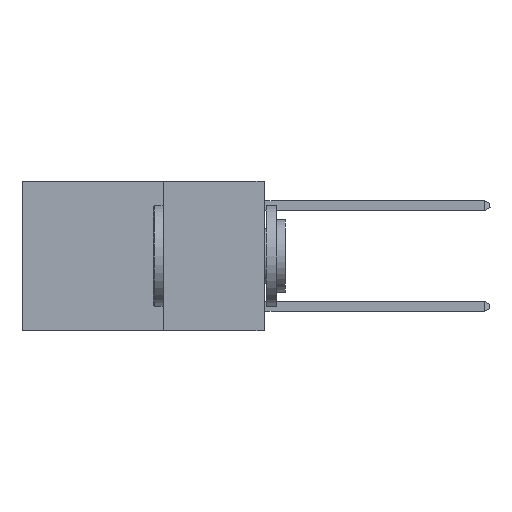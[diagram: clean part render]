
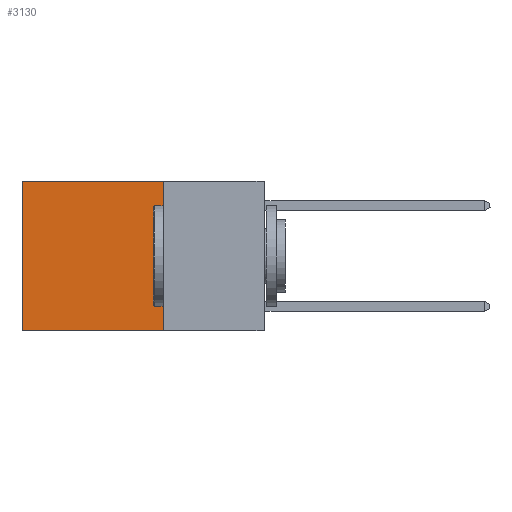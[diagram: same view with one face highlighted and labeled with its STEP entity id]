
A CAD part, left-side view. The second image highlights one B-rep face of the part: STEP entity #3130.
In plain terms, the highlighted planar face has unit normal (-1, 0, 0).
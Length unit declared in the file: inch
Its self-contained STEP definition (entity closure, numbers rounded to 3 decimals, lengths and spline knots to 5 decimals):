
#243 = VERTEX_POINT ( 'NONE', #12224 ) ;
#468 = DIRECTION ( 'NONE',  ( 0., 1., 0. ) ) ;
#2147 = PLANE ( 'NONE',  #14639 ) ;
#3090 = ORIENTED_EDGE ( 'NONE', *, *, #7713, .F. ) ;
#3130 = ADVANCED_FACE ( 'NONE', ( #13995 ), #2147, .F. ) ;
#3532 = ORIENTED_EDGE ( 'NONE', *, *, #5945, .T. ) ;
#3566 = DIRECTION ( 'NONE',  ( 1., 0., 0. ) ) ;
#4046 = LINE ( 'NONE', #7949, #10388 ) ;
#4439 = CARTESIAN_POINT ( 'NONE',  ( 0.2625, 0.6, 0. ) ) ;
#4689 = LINE ( 'NONE', #11690, #8244 ) ;
#5429 = EDGE_CURVE ( 'NONE', #16957, #13461, #14746, .T. ) ;
#5945 = EDGE_CURVE ( 'NONE', #243, #14178, #10211, .T. ) ;
#7367 = ORIENTED_EDGE ( 'NONE', *, *, #11386, .T. ) ;
#7713 = EDGE_CURVE ( 'NONE', #243, #16957, #4046, .T. ) ;
#7949 = CARTESIAN_POINT ( 'NONE',  ( 0.2625, 0.25, 0. ) ) ;
#8244 = VECTOR ( 'NONE', #14406, 39.37008 ) ;
#8345 = VECTOR ( 'NONE', #17150, 39.37008 ) ;
#9027 = ORIENTED_EDGE ( 'NONE', *, *, #5429, .F. ) ;
#9803 = VECTOR ( 'NONE', #468, 39.37008 ) ;
#10211 = LINE ( 'NONE', #11398, #9803 ) ;
#10388 = VECTOR ( 'NONE', #10649, 39.37008 ) ;
#10636 = CARTESIAN_POINT ( 'NONE',  ( 0.2625, 0.25, -0.37 ) ) ;
#10649 = DIRECTION ( 'NONE',  ( 0., 0., -1. ) ) ;
#10768 = EDGE_LOOP ( 'NONE', ( #7367, #9027, #3090, #3532 ) ) ;
#11386 = EDGE_CURVE ( 'NONE', #14178, #13461, #4689, .T. ) ;
#11398 = CARTESIAN_POINT ( 'NONE',  ( 0.2625, 0.25, 0. ) ) ;
#11657 = CARTESIAN_POINT ( 'NONE',  ( 0.2625, 0.25, -0.37 ) ) ;
#11684 = CARTESIAN_POINT ( 'NONE',  ( 0.2625, 0.25, 0. ) ) ;
#11690 = CARTESIAN_POINT ( 'NONE',  ( 0.2625, 0.6, 0. ) ) ;
#12224 = CARTESIAN_POINT ( 'NONE',  ( 0.2625, 0.25, 0. ) ) ;
#13095 = DIRECTION ( 'NONE',  ( 0., 0., -1. ) ) ;
#13461 = VERTEX_POINT ( 'NONE', #16589 ) ;
#13995 = FACE_OUTER_BOUND ( 'NONE', #10768, .T. ) ;
#14178 = VERTEX_POINT ( 'NONE', #4439 ) ;
#14406 = DIRECTION ( 'NONE',  ( 0., 0., -1. ) ) ;
#14639 = AXIS2_PLACEMENT_3D ( 'NONE', #11684, #3566, #13095 ) ;
#14746 = LINE ( 'NONE', #11657, #8345 ) ;
#16589 = CARTESIAN_POINT ( 'NONE',  ( 0.2625, 0.6, -0.37 ) ) ;
#16957 = VERTEX_POINT ( 'NONE', #10636 ) ;
#17150 = DIRECTION ( 'NONE',  ( 0., 1., 0. ) ) ;
